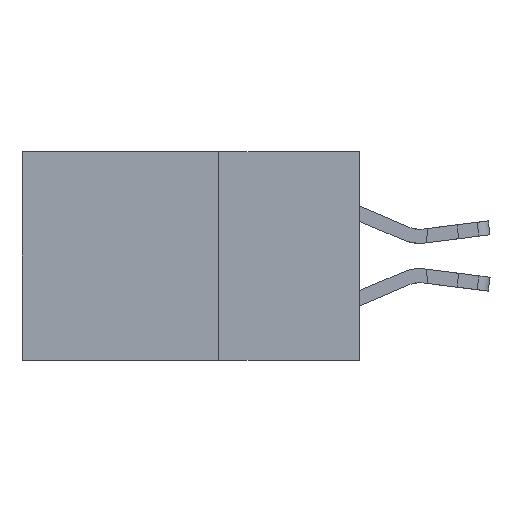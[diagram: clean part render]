
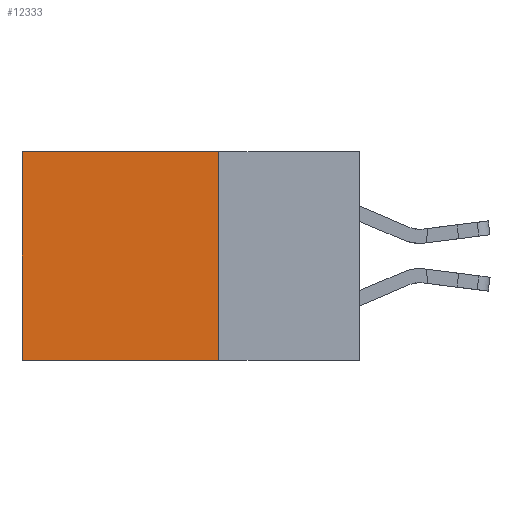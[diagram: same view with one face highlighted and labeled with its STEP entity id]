
A CAD part, left-side view. The second image highlights one B-rep face of the part: STEP entity #12333.
In plain terms, the highlighted planar face has unit normal (-1, 0, 0).
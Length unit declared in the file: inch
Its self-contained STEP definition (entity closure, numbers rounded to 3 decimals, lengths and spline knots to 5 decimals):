
#509 = ORIENTED_EDGE ( 'NONE', *, *, #10599, .T. ) ;
#579 = CARTESIAN_POINT ( 'NONE',  ( 0.2875, 0.6, 0. ) ) ;
#1152 = CARTESIAN_POINT ( 'NONE',  ( 0.2875, 0.6, 0. ) ) ;
#1835 = FACE_OUTER_BOUND ( 'NONE', #12363, .T. ) ;
#3350 = EDGE_CURVE ( 'NONE', #29311, #28997, #15119, .T. ) ;
#5442 = VECTOR ( 'NONE', #30778, 39.37008 ) ;
#7156 = DIRECTION ( 'NONE',  ( 0., 1., 0. ) ) ;
#8608 = DIRECTION ( 'NONE',  ( 0., 0., -1. ) ) ;
#9139 = VERTEX_POINT ( 'NONE', #24631 ) ;
#9192 = VECTOR ( 'NONE', #8608, 39.37008 ) ;
#9581 = PLANE ( 'NONE',  #17985 ) ;
#10599 = EDGE_CURVE ( 'NONE', #23762, #9139, #11443, .T. ) ;
#10699 = ORIENTED_EDGE ( 'NONE', *, *, #31149, .T. ) ;
#11115 = DIRECTION ( 'NONE',  ( 0., 0., -1. ) ) ;
#11443 = LINE ( 'NONE', #1152, #24833 ) ;
#12333 = ADVANCED_FACE ( 'NONE', ( #1835 ), #9581, .F. ) ;
#12363 = EDGE_LOOP ( 'NONE', ( #509, #16020, #29808, #10699 ) ) ;
#14674 = DIRECTION ( 'NONE',  ( 0., 0., -1. ) ) ;
#14783 = LINE ( 'NONE', #22163, #32490 ) ;
#15119 = LINE ( 'NONE', #20777, #9192 ) ;
#16020 = ORIENTED_EDGE ( 'NONE', *, *, #16293, .F. ) ;
#16293 = EDGE_CURVE ( 'NONE', #28997, #9139, #14783, .T. ) ;
#17985 = AXIS2_PLACEMENT_3D ( 'NONE', #27195, #27311, #14674 ) ;
#20777 = CARTESIAN_POINT ( 'NONE',  ( 0.2875, 0.25, 0. ) ) ;
#22163 = CARTESIAN_POINT ( 'NONE',  ( 0.2875, 0.25, -0.37 ) ) ;
#23762 = VERTEX_POINT ( 'NONE', #579 ) ;
#23990 = LINE ( 'NONE', #30455, #5442 ) ;
#24631 = CARTESIAN_POINT ( 'NONE',  ( 0.2875, 0.6, -0.37 ) ) ;
#24833 = VECTOR ( 'NONE', #11115, 39.37008 ) ;
#27195 = CARTESIAN_POINT ( 'NONE',  ( 0.2875, 0.25, 0. ) ) ;
#27311 = DIRECTION ( 'NONE',  ( 1., 0., 0. ) ) ;
#28963 = CARTESIAN_POINT ( 'NONE',  ( 0.2875, 0.25, -0.37 ) ) ;
#28997 = VERTEX_POINT ( 'NONE', #28963 ) ;
#29311 = VERTEX_POINT ( 'NONE', #32244 ) ;
#29808 = ORIENTED_EDGE ( 'NONE', *, *, #3350, .F. ) ;
#30455 = CARTESIAN_POINT ( 'NONE',  ( 0.2875, 0.25, 0. ) ) ;
#30778 = DIRECTION ( 'NONE',  ( 0., 1., 0. ) ) ;
#31149 = EDGE_CURVE ( 'NONE', #29311, #23762, #23990, .T. ) ;
#32244 = CARTESIAN_POINT ( 'NONE',  ( 0.2875, 0.25, 0. ) ) ;
#32490 = VECTOR ( 'NONE', #7156, 39.37008 ) ;
